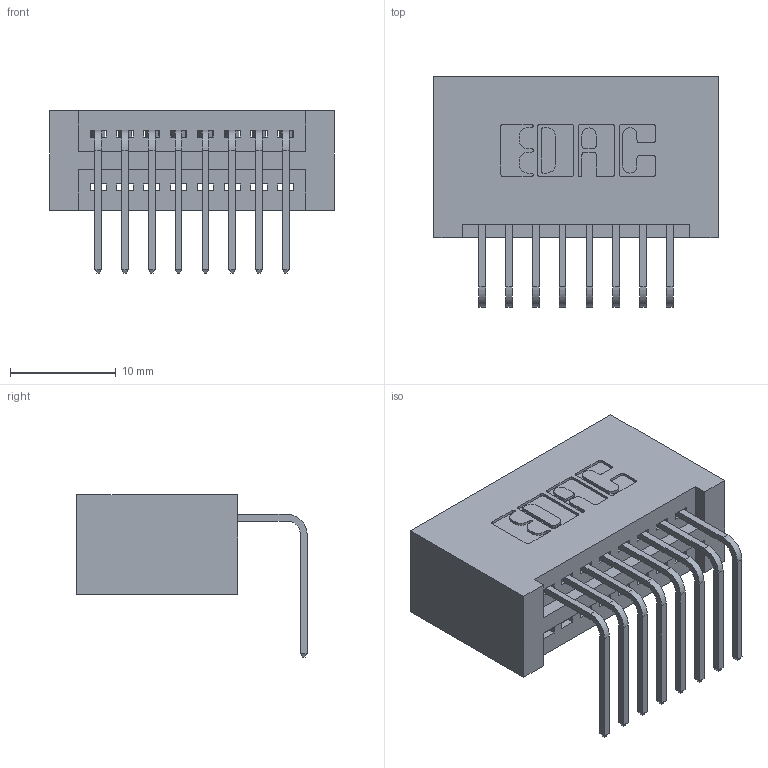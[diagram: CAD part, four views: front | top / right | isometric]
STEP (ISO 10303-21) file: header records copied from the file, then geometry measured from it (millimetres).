
FILE_DESCRIPTION (( 'STEP AP203' ), '1' );
FILE_NAME ('345-008-558-101.STEP', '2019-10-10T11:04:13', ( '' ), ( '' ), 'SwSTEP 2.0', 'SolidWorks 2016', '' );
FILE_SCHEMA (( 'CONFIG_CONTROL_DESIGN' ));
Length unit declared in the file: inch
Products named in the file (3): 345 Part_No Mounting Lugs; 345-292-001_558 Tail - 2; 345-008-558-101
Assembly tree (9 placements, depth 2):
  345-008-558-101
    345 Part_No Mounting Lugs
    345-292-001_558 Tail - 2  x8
Bounding box: 26.92 x 21.83 x 15.37 mm (x, y, z)
Volume: 2889.8 mm3; surface area: 3724.9 mm2
Topology: 9 solids, 9 shells, 598 faces, 1773 edges, 1170 vertices
Faces by surface type: plane 412, cylinder 186
Entity records: 10405 total; most frequent: CARTESIAN_POINT 1812, ORIENTED_EDGE 1754, DIRECTION 1625, EDGE_CURVE 877, VECTOR 721, LINE 721, VERTEX_POINT 582, AXIS2_PLACEMENT_3D 452
